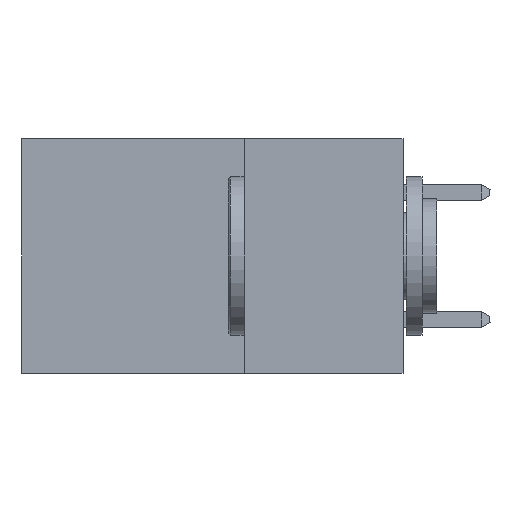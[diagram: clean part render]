
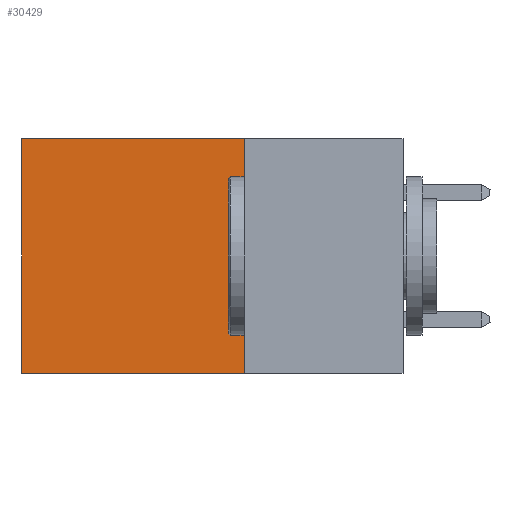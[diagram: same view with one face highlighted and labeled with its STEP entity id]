
A CAD part, left-side view. The second image highlights one B-rep face of the part: STEP entity #30429.
In plain terms, the highlighted planar face has unit normal (-1, 0, 0).
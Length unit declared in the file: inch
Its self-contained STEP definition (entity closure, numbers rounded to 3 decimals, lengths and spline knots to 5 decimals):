
#1345 = CARTESIAN_POINT ( 'NONE',  ( 0.2875, 0.6, 0. ) ) ;
#2296 = DIRECTION ( 'NONE',  ( 0., 0., -1. ) ) ;
#3855 = VERTEX_POINT ( 'NONE', #25584 ) ;
#4154 = CARTESIAN_POINT ( 'NONE',  ( 0.2875, 0.25, 0. ) ) ;
#4715 = LINE ( 'NONE', #19792, #39756 ) ;
#5005 = EDGE_CURVE ( 'NONE', #25448, #17096, #6835, .T. ) ;
#6835 = LINE ( 'NONE', #11686, #23287 ) ;
#8362 = DIRECTION ( 'NONE',  ( 0., 0., -1. ) ) ;
#8436 = DIRECTION ( 'NONE',  ( 0., 1., 0. ) ) ;
#9146 = CARTESIAN_POINT ( 'NONE',  ( 0.2875, 0.25, 0. ) ) ;
#10443 = ORIENTED_EDGE ( 'NONE', *, *, #14570, .F. ) ;
#11686 = CARTESIAN_POINT ( 'NONE',  ( 0.2875, 0.25, 0. ) ) ;
#12530 = VERTEX_POINT ( 'NONE', #22171 ) ;
#12977 = LINE ( 'NONE', #9146, #23883 ) ;
#13141 = CARTESIAN_POINT ( 'NONE',  ( 0.2875, 0.25, 0. ) ) ;
#14570 = EDGE_CURVE ( 'NONE', #12530, #3855, #4715, .T. ) ;
#15994 = ORIENTED_EDGE ( 'NONE', *, *, #5005, .T. ) ;
#16048 = FACE_OUTER_BOUND ( 'NONE', #17855, .T. ) ;
#17096 = VERTEX_POINT ( 'NONE', #26417 ) ;
#17855 = EDGE_LOOP ( 'NONE', ( #30625, #10443, #31352, #15994 ) ) ;
#18070 = DIRECTION ( 'NONE',  ( 1., 0., 0. ) ) ;
#19792 = CARTESIAN_POINT ( 'NONE',  ( 0.2875, 0.25, -0.37 ) ) ;
#22171 = CARTESIAN_POINT ( 'NONE',  ( 0.2875, 0.25, -0.37 ) ) ;
#22201 = DIRECTION ( 'NONE',  ( 0., 0., -1. ) ) ;
#23287 = VECTOR ( 'NONE', #8436, 39.37008 ) ;
#23883 = VECTOR ( 'NONE', #2296, 39.37008 ) ;
#25448 = VERTEX_POINT ( 'NONE', #13141 ) ;
#25584 = CARTESIAN_POINT ( 'NONE',  ( 0.2875, 0.6, -0.37 ) ) ;
#26417 = CARTESIAN_POINT ( 'NONE',  ( 0.2875, 0.6, 0. ) ) ;
#27417 = DIRECTION ( 'NONE',  ( 0., 1., 0. ) ) ;
#28860 = EDGE_CURVE ( 'NONE', #25448, #12530, #12977, .T. ) ;
#30429 = ADVANCED_FACE ( 'NONE', ( #16048 ), #32477, .F. ) ;
#30625 = ORIENTED_EDGE ( 'NONE', *, *, #35810, .T. ) ;
#31352 = ORIENTED_EDGE ( 'NONE', *, *, #28860, .F. ) ;
#31724 = LINE ( 'NONE', #1345, #33874 ) ;
#32477 = PLANE ( 'NONE',  #43496 ) ;
#33874 = VECTOR ( 'NONE', #8362, 39.37008 ) ;
#35810 = EDGE_CURVE ( 'NONE', #17096, #3855, #31724, .T. ) ;
#39756 = VECTOR ( 'NONE', #27417, 39.37008 ) ;
#43496 = AXIS2_PLACEMENT_3D ( 'NONE', #4154, #18070, #22201 ) ;
